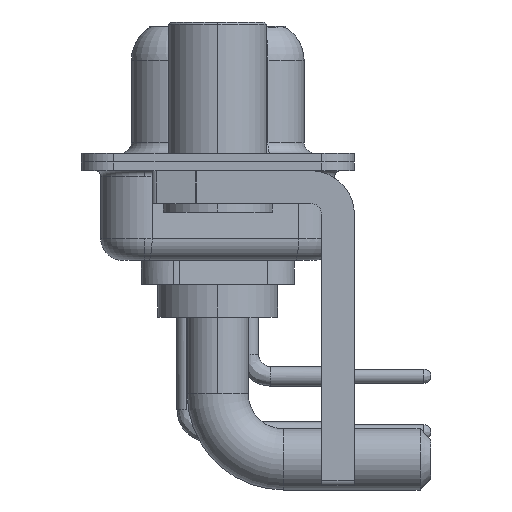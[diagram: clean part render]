
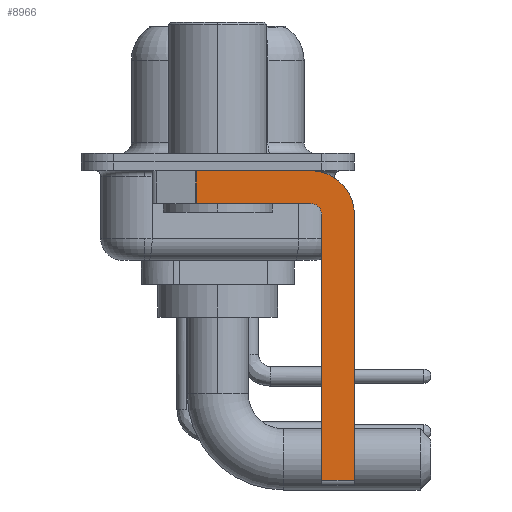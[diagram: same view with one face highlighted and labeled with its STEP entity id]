
A CAD part, left-side view. The second image highlights one B-rep face of the part: STEP entity #8966.
In plain terms, the highlighted planar face has unit normal (-1, 0, 0).
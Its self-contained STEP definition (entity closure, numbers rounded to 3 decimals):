
#22 = CARTESIAN_POINT ( 'NONE',  ( -2.9, 0.978, -1.9 ) ) ;
#88 = VECTOR ( 'NONE', #13733, 1000. ) ;
#91 = AXIS2_PLACEMENT_3D ( 'NONE', #8714, #733, #18704 ) ;
#122 = EDGE_LOOP ( 'NONE', ( #20236, #9742, #9483, #14690, #22155, #2846, #3827, #10378 ) ) ;
#430 = EDGE_CURVE ( 'NONE', #21086, #18625, #17530, .T. ) ;
#526 = AXIS2_PLACEMENT_3D ( 'NONE', #18918, #25050, #4927 ) ;
#658 = VERTEX_POINT ( 'NONE', #24552 ) ;
#733 = DIRECTION ( 'NONE',  ( -1., 0., 0. ) ) ;
#1126 = EDGE_CURVE ( 'NONE', #658, #24405, #9478, .T. ) ;
#1704 = LINE ( 'NONE', #9688, #19972 ) ;
#2680 = FACE_OUTER_BOUND ( 'NONE', #122, .T. ) ;
#2846 = ORIENTED_EDGE ( 'NONE', *, *, #14139, .T. ) ;
#3392 = LINE ( 'NONE', #23238, #6386 ) ;
#3758 = DIRECTION ( 'NONE',  ( 0., -1., 0. ) ) ;
#3827 = ORIENTED_EDGE ( 'NONE', *, *, #9762, .F. ) ;
#4221 = EDGE_CURVE ( 'NONE', #17721, #6735, #19872, .T. ) ;
#4340 = DIRECTION ( 'NONE',  ( 0., 0., -1. ) ) ;
#4554 = EDGE_CURVE ( 'NONE', #18625, #24405, #3392, .T. ) ;
#4789 = CARTESIAN_POINT ( 'NONE',  ( -2.9, -4.75, -2.4 ) ) ;
#4927 = DIRECTION ( 'NONE',  ( 0., 0., -1. ) ) ;
#5602 = CARTESIAN_POINT ( 'NONE',  ( -2.9, 3., -0.4 ) ) ;
#5666 = DIRECTION ( 'NONE',  ( 1., 0., 0. ) ) ;
#5690 = DIRECTION ( 'NONE',  ( 0., 0., 1. ) ) ;
#5787 = CARTESIAN_POINT ( 'NONE',  ( -2.9, -6.25, -14.55 ) ) ;
#5799 = CARTESIAN_POINT ( 'NONE',  ( -2.9, -4.25, -2.4 ) ) ;
#6248 = AXIS2_PLACEMENT_3D ( 'NONE', #5799, #5666, #8202 ) ;
#6386 = VECTOR ( 'NONE', #13371, 1000. ) ;
#6735 = VERTEX_POINT ( 'NONE', #18739 ) ;
#7296 = EDGE_CURVE ( 'NONE', #658, #17721, #13466, .T. ) ;
#7489 = VECTOR ( 'NONE', #7533, 1000. ) ;
#7533 = DIRECTION ( 'NONE',  ( 0., -1., 0. ) ) ;
#8202 = DIRECTION ( 'NONE',  ( 0., 0., -1. ) ) ;
#8211 = VECTOR ( 'NONE', #3758, 1000. ) ;
#8640 = VERTEX_POINT ( 'NONE', #21641 ) ;
#8714 = CARTESIAN_POINT ( 'NONE',  ( -2.9, -4.25, -2.4 ) ) ;
#8966 = ADVANCED_FACE ( 'NONE', ( #2680 ), #20916, .F. ) ;
#9478 = LINE ( 'NONE', #22, #88 ) ;
#9483 = ORIENTED_EDGE ( 'NONE', *, *, #4554, .F. ) ;
#9688 = CARTESIAN_POINT ( 'NONE',  ( -2.9, -4.75, -14.8 ) ) ;
#9742 = ORIENTED_EDGE ( 'NONE', *, *, #1126, .T. ) ;
#9762 = EDGE_CURVE ( 'NONE', #6735, #22788, #14993, .T. ) ;
#10378 = ORIENTED_EDGE ( 'NONE', *, *, #4221, .F. ) ;
#12576 = CARTESIAN_POINT ( 'NONE',  ( -2.9, -4.25, -1.9 ) ) ;
#13371 = DIRECTION ( 'NONE',  ( 0., 1., 0. ) ) ;
#13466 = LINE ( 'NONE', #5602, #8211 ) ;
#13733 = DIRECTION ( 'NONE',  ( 0., 0., -1. ) ) ;
#14139 = EDGE_CURVE ( 'NONE', #8640, #22788, #19919, .T. ) ;
#14590 = CARTESIAN_POINT ( 'NONE',  ( -2.9, -6.25, -2.4 ) ) ;
#14642 = CARTESIAN_POINT ( 'NONE',  ( -2.9, -4.25, -0.4 ) ) ;
#14690 = ORIENTED_EDGE ( 'NONE', *, *, #430, .F. ) ;
#14993 = LINE ( 'NONE', #14590, #23500 ) ;
#15387 = CARTESIAN_POINT ( 'NONE',  ( -2.9, -4.25, -14.55 ) ) ;
#17530 = CIRCLE ( 'NONE', #91, 0.5 ) ;
#17721 = VERTEX_POINT ( 'NONE', #14642 ) ;
#18625 = VERTEX_POINT ( 'NONE', #12576 ) ;
#18704 = DIRECTION ( 'NONE',  ( 0., 0., 1. ) ) ;
#18739 = CARTESIAN_POINT ( 'NONE',  ( -2.9, -6.25, -2.4 ) ) ;
#18918 = CARTESIAN_POINT ( 'NONE',  ( -2.9, -4.25, -2.4 ) ) ;
#19872 = CIRCLE ( 'NONE', #6248, 2. ) ;
#19919 = LINE ( 'NONE', #15387, #7489 ) ;
#19972 = VECTOR ( 'NONE', #5690, 1000. ) ;
#20236 = ORIENTED_EDGE ( 'NONE', *, *, #7296, .F. ) ;
#20916 = PLANE ( 'NONE',  #526 ) ;
#21086 = VERTEX_POINT ( 'NONE', #4789 ) ;
#21641 = CARTESIAN_POINT ( 'NONE',  ( -2.9, -4.75, -14.55 ) ) ;
#22155 = ORIENTED_EDGE ( 'NONE', *, *, #23247, .F. ) ;
#22509 = CARTESIAN_POINT ( 'NONE',  ( -2.9, 0.978, -1.9 ) ) ;
#22788 = VERTEX_POINT ( 'NONE', #5787 ) ;
#23238 = CARTESIAN_POINT ( 'NONE',  ( -2.9, -4.25, -1.9 ) ) ;
#23247 = EDGE_CURVE ( 'NONE', #8640, #21086, #1704, .T. ) ;
#23500 = VECTOR ( 'NONE', #4340, 1000. ) ;
#24405 = VERTEX_POINT ( 'NONE', #22509 ) ;
#24552 = CARTESIAN_POINT ( 'NONE',  ( -2.9, 0.978, -0.4 ) ) ;
#25050 = DIRECTION ( 'NONE',  ( 1., 0., 0. ) ) ;
